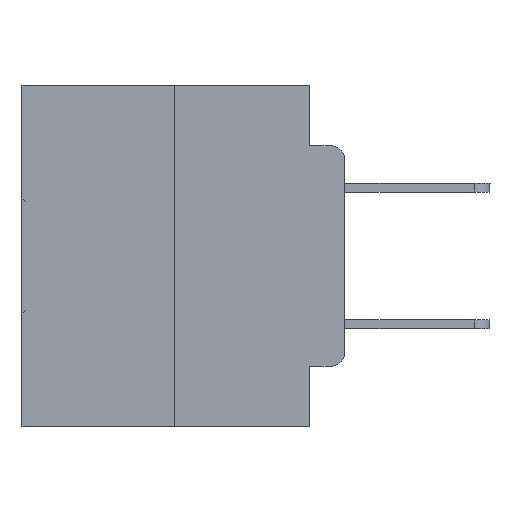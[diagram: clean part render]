
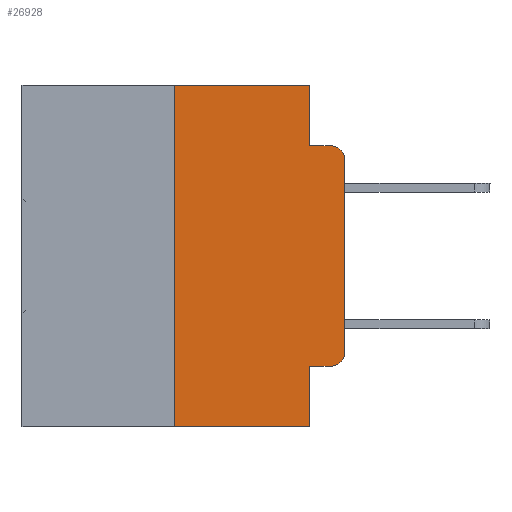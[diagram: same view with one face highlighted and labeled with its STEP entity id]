
A CAD part, left-side view. The second image highlights one B-rep face of the part: STEP entity #26928.
In plain terms, the highlighted planar face has unit normal (-1, 0, 0).
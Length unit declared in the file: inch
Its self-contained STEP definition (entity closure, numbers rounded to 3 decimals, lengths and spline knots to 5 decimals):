
#630 = VECTOR ( 'NONE', #8281, 39.37008 ) ;
#859 = VECTOR ( 'NONE', #3970, 39.37008 ) ;
#1061 = CIRCLE ( 'NONE', #8487, 0.02 ) ;
#1173 = DIRECTION ( 'NONE',  ( 1., 0., 0. ) ) ;
#1957 = VECTOR ( 'NONE', #13263, 39.37008 ) ;
#2657 = ORIENTED_EDGE ( 'NONE', *, *, #17315, .F. ) ;
#2947 = CARTESIAN_POINT ( 'NONE',  ( 0., 0.25, -0.5 ) ) ;
#3050 = ORIENTED_EDGE ( 'NONE', *, *, #6292, .F. ) ;
#3697 = LINE ( 'NONE', #12375, #10388 ) ;
#3970 = DIRECTION ( 'NONE',  ( 0., -1., 0. ) ) ;
#4778 = DIRECTION ( 'NONE',  ( 0., -1., 0. ) ) ;
#5691 = FACE_OUTER_BOUND ( 'NONE', #29283, .T. ) ;
#5799 = EDGE_CURVE ( 'NONE', #23322, #24986, #20692, .T. ) ;
#5917 = VERTEX_POINT ( 'NONE', #2947 ) ;
#6292 = EDGE_CURVE ( 'NONE', #14102, #23737, #26412, .T. ) ;
#6952 = CARTESIAN_POINT ( 'NONE',  ( 0., 0.051, 0. ) ) ;
#7117 = EDGE_CURVE ( 'NONE', #5917, #18446, #7633, .T. ) ;
#7511 = ORIENTED_EDGE ( 'NONE', *, *, #14085, .T. ) ;
#7611 = DIRECTION ( 'NONE',  ( -1., 0., 0. ) ) ;
#7633 = LINE ( 'NONE', #13869, #859 ) ;
#7882 = CARTESIAN_POINT ( 'NONE',  ( 0., 0.051, -0.0885 ) ) ;
#8281 = DIRECTION ( 'NONE',  ( 0., 0., -1. ) ) ;
#8323 = CARTESIAN_POINT ( 'NONE',  ( 0., 0.051, -0.4115 ) ) ;
#8487 = AXIS2_PLACEMENT_3D ( 'NONE', #10682, #27736, #13144 ) ;
#9104 = LINE ( 'NONE', #7882, #14841 ) ;
#9151 = VECTOR ( 'NONE', #31797, 39.37008 ) ;
#9935 = VERTEX_POINT ( 'NONE', #15086 ) ;
#10388 = VECTOR ( 'NONE', #26950, 39.37008 ) ;
#10435 = CARTESIAN_POINT ( 'NONE',  ( 0., 0., -0.3915 ) ) ;
#10585 = ORIENTED_EDGE ( 'NONE', *, *, #27150, .F. ) ;
#10682 = CARTESIAN_POINT ( 'NONE',  ( 0., 0.02, -0.1085 ) ) ;
#11929 = AXIS2_PLACEMENT_3D ( 'NONE', #23331, #1173, #18485 ) ;
#12297 = EDGE_CURVE ( 'NONE', #24986, #9935, #15645, .T. ) ;
#12375 = CARTESIAN_POINT ( 'NONE',  ( 0., 0.25, 0. ) ) ;
#13144 = DIRECTION ( 'NONE',  ( 0., 0., -1. ) ) ;
#13181 = LINE ( 'NONE', #17964, #630 ) ;
#13263 = DIRECTION ( 'NONE',  ( 0., -1., 0. ) ) ;
#13447 = VECTOR ( 'NONE', #4778, 39.37008 ) ;
#13869 = CARTESIAN_POINT ( 'NONE',  ( 0., 0.473, -0.5 ) ) ;
#13910 = ORIENTED_EDGE ( 'NONE', *, *, #28769, .F. ) ;
#14085 = EDGE_CURVE ( 'NONE', #27451, #23322, #21652, .T. ) ;
#14102 = VERTEX_POINT ( 'NONE', #27950 ) ;
#14419 = CARTESIAN_POINT ( 'NONE',  ( 0., 0.02, -0.4115 ) ) ;
#14680 = ORIENTED_EDGE ( 'NONE', *, *, #30441, .T. ) ;
#14841 = VECTOR ( 'NONE', #29873, 39.37008 ) ;
#15086 = CARTESIAN_POINT ( 'NONE',  ( 0., 0., -0.1085 ) ) ;
#15126 = ORIENTED_EDGE ( 'NONE', *, *, #12297, .T. ) ;
#15645 = LINE ( 'NONE', #24430, #9151 ) ;
#15718 = EDGE_CURVE ( 'NONE', #27451, #18446, #13181, .T. ) ;
#16805 = DIRECTION ( 'NONE',  ( 0., 0., -1. ) ) ;
#17315 = EDGE_CURVE ( 'NONE', #5917, #14102, #3697, .T. ) ;
#17964 = CARTESIAN_POINT ( 'NONE',  ( 0., 0.051, 0. ) ) ;
#18446 = VERTEX_POINT ( 'NONE', #30934 ) ;
#18485 = DIRECTION ( 'NONE',  ( 0., 0., -1. ) ) ;
#18837 = CARTESIAN_POINT ( 'NONE',  ( 0., 0.051, 0. ) ) ;
#20692 = CIRCLE ( 'NONE', #24585, 0.02 ) ;
#21652 = LINE ( 'NONE', #8323, #1957 ) ;
#21725 = CARTESIAN_POINT ( 'NONE',  ( 0., 0.051, -0.0885 ) ) ;
#22236 = CARTESIAN_POINT ( 'NONE',  ( 0., 0.02, -0.3915 ) ) ;
#23322 = VERTEX_POINT ( 'NONE', #14419 ) ;
#23331 = CARTESIAN_POINT ( 'NONE',  ( 0., 0.473, 0. ) ) ;
#23336 = VECTOR ( 'NONE', #16805, 39.37008 ) ;
#23737 = VERTEX_POINT ( 'NONE', #18837 ) ;
#23750 = CARTESIAN_POINT ( 'NONE',  ( 0., 0.02, -0.0885 ) ) ;
#23853 = VERTEX_POINT ( 'NONE', #21725 ) ;
#24430 = CARTESIAN_POINT ( 'NONE',  ( 0., 0., 0. ) ) ;
#24585 = AXIS2_PLACEMENT_3D ( 'NONE', #22236, #7611, #24704 ) ;
#24704 = DIRECTION ( 'NONE',  ( 0., 0., -1. ) ) ;
#24986 = VERTEX_POINT ( 'NONE', #10435 ) ;
#26412 = LINE ( 'NONE', #26890, #13447 ) ;
#26865 = ORIENTED_EDGE ( 'NONE', *, *, #15718, .F. ) ;
#26890 = CARTESIAN_POINT ( 'NONE',  ( 0., 0.473, 0. ) ) ;
#26928 = ADVANCED_FACE ( 'NONE', ( #5691 ), #30688, .F. ) ;
#26950 = DIRECTION ( 'NONE',  ( 0., 0., 1. ) ) ;
#27150 = EDGE_CURVE ( 'NONE', #23737, #23853, #30593, .T. ) ;
#27401 = ORIENTED_EDGE ( 'NONE', *, *, #5799, .T. ) ;
#27451 = VERTEX_POINT ( 'NONE', #27584 ) ;
#27584 = CARTESIAN_POINT ( 'NONE',  ( 0., 0.051, -0.4115 ) ) ;
#27736 = DIRECTION ( 'NONE',  ( -1., 0., 0. ) ) ;
#27950 = CARTESIAN_POINT ( 'NONE',  ( 0., 0.25, 0. ) ) ;
#28769 = EDGE_CURVE ( 'NONE', #23853, #31186, #9104, .T. ) ;
#29283 = EDGE_LOOP ( 'NONE', ( #15126, #14680, #13910, #10585, #3050, #2657, #30055, #26865, #7511, #27401 ) ) ;
#29873 = DIRECTION ( 'NONE',  ( 0., -1., 0. ) ) ;
#30055 = ORIENTED_EDGE ( 'NONE', *, *, #7117, .T. ) ;
#30441 = EDGE_CURVE ( 'NONE', #9935, #31186, #1061, .T. ) ;
#30593 = LINE ( 'NONE', #6952, #23336 ) ;
#30688 = PLANE ( 'NONE',  #11929 ) ;
#30934 = CARTESIAN_POINT ( 'NONE',  ( 0., 0.051, -0.5 ) ) ;
#31186 = VERTEX_POINT ( 'NONE', #23750 ) ;
#31797 = DIRECTION ( 'NONE',  ( 0., 0., 1. ) ) ;
